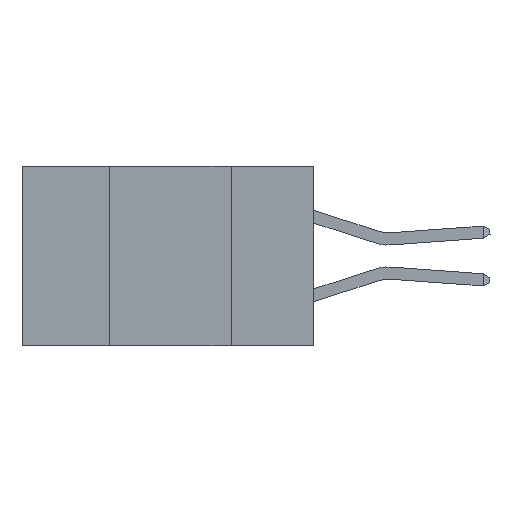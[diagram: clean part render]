
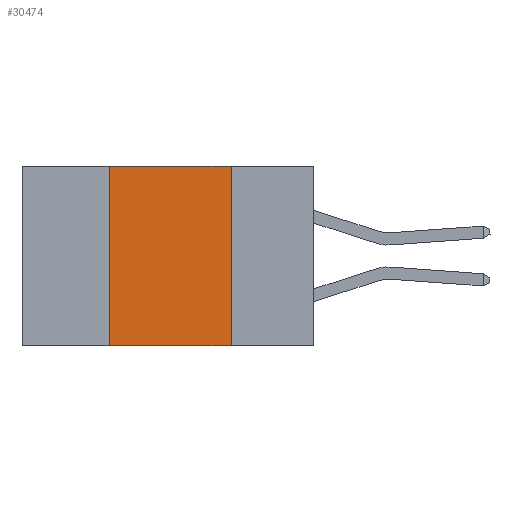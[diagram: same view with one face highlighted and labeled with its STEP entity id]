
A CAD part, left-side view. The second image highlights one B-rep face of the part: STEP entity #30474.
In plain terms, the highlighted planar face has unit normal (-1, 0, 0).
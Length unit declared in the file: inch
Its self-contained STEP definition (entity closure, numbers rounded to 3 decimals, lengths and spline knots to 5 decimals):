
#99 = EDGE_CURVE ( 'NONE', #18082, #4847, #8106, .T. ) ;
#4847 = VERTEX_POINT ( 'NONE', #31423 ) ;
#5069 = DIRECTION ( 'NONE',  ( 0., 0., -1. ) ) ;
#6651 = DIRECTION ( 'NONE',  ( 0., 0., 1. ) ) ;
#7697 = DIRECTION ( 'NONE',  ( 0., -1., 0. ) ) ;
#8106 = LINE ( 'NONE', #14790, #21617 ) ;
#8113 = ORIENTED_EDGE ( 'NONE', *, *, #33057, .F. ) ;
#8449 = EDGE_CURVE ( 'NONE', #12055, #16140, #20424, .T. ) ;
#12055 = VERTEX_POINT ( 'NONE', #27421 ) ;
#12708 = DIRECTION ( 'NONE',  ( 1., 0., 0. ) ) ;
#14790 = CARTESIAN_POINT ( 'NONE',  ( 0., 0.6, -0.37 ) ) ;
#15695 = EDGE_CURVE ( 'NONE', #18082, #12055, #32993, .T. ) ;
#15818 = VECTOR ( 'NONE', #5069, 39.37008 ) ;
#16140 = VERTEX_POINT ( 'NONE', #33333 ) ;
#16424 = EDGE_LOOP ( 'NONE', ( #8113, #17009, #18672, #20350 ) ) ;
#16881 = CARTESIAN_POINT ( 'NONE',  ( 0., 0.42, -0.37 ) ) ;
#17009 = ORIENTED_EDGE ( 'NONE', *, *, #8449, .F. ) ;
#17294 = AXIS2_PLACEMENT_3D ( 'NONE', #28861, #12708, #31554 ) ;
#18082 = VERTEX_POINT ( 'NONE', #16881 ) ;
#18668 = VECTOR ( 'NONE', #6651, 39.37008 ) ;
#18672 = ORIENTED_EDGE ( 'NONE', *, *, #15695, .F. ) ;
#20350 = ORIENTED_EDGE ( 'NONE', *, *, #99, .T. ) ;
#20424 = LINE ( 'NONE', #21004, #32219 ) ;
#20717 = PLANE ( 'NONE',  #17294 ) ;
#21004 = CARTESIAN_POINT ( 'NONE',  ( 0., 0.6, 0. ) ) ;
#21226 = CARTESIAN_POINT ( 'NONE',  ( 0., 0.17, 0. ) ) ;
#21482 = FACE_OUTER_BOUND ( 'NONE', #16424, .T. ) ;
#21617 = VECTOR ( 'NONE', #29312, 39.37008 ) ;
#22128 = LINE ( 'NONE', #21226, #15818 ) ;
#22800 = CARTESIAN_POINT ( 'NONE',  ( 0., 0.42, 0. ) ) ;
#27421 = CARTESIAN_POINT ( 'NONE',  ( 0., 0.42, 0. ) ) ;
#28861 = CARTESIAN_POINT ( 'NONE',  ( 0., 0.6, 0. ) ) ;
#29312 = DIRECTION ( 'NONE',  ( 0., -1., 0. ) ) ;
#30474 = ADVANCED_FACE ( 'NONE', ( #21482 ), #20717, .F. ) ;
#31423 = CARTESIAN_POINT ( 'NONE',  ( 0., 0.17, -0.37 ) ) ;
#31554 = DIRECTION ( 'NONE',  ( 0., 0., -1. ) ) ;
#32219 = VECTOR ( 'NONE', #7697, 39.37008 ) ;
#32993 = LINE ( 'NONE', #22800, #18668 ) ;
#33057 = EDGE_CURVE ( 'NONE', #16140, #4847, #22128, .T. ) ;
#33333 = CARTESIAN_POINT ( 'NONE',  ( 0., 0.17, 0. ) ) ;
